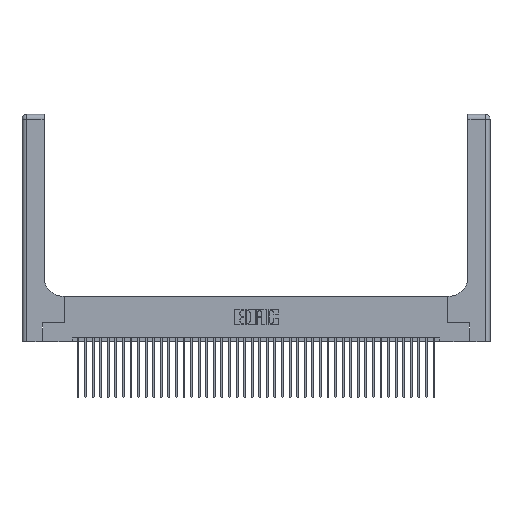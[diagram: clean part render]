
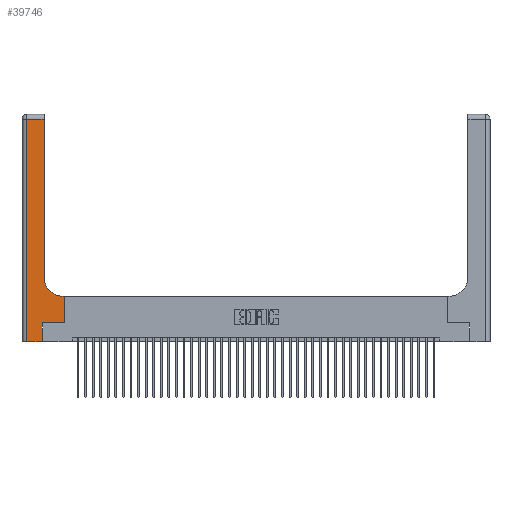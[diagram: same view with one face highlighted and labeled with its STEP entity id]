
A CAD part, top view. The second image highlights one B-rep face of the part: STEP entity #39746.
In plain terms, the highlighted planar face has unit normal (0, 0, 1).
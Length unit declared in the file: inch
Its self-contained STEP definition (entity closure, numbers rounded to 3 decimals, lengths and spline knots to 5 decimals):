
#254 = ORIENTED_EDGE ( 'NONE', *, *, #15014, .T. ) ;
#585 = CARTESIAN_POINT ( 'NONE',  ( 0., 0., 0.37 ) ) ;
#1194 = VERTEX_POINT ( 'NONE', #22436 ) ;
#1436 = LINE ( 'NONE', #27474, #26278 ) ;
#3791 = VERTEX_POINT ( 'NONE', #14060 ) ;
#3934 = CARTESIAN_POINT ( 'NONE',  ( 0.269, 0., 0.37 ) ) ;
#5589 = VERTEX_POINT ( 'NONE', #40948 ) ;
#5886 = VECTOR ( 'NONE', #22582, 39.37008 ) ;
#6122 = VECTOR ( 'NONE', #21281, 39.37008 ) ;
#7618 = AXIS2_PLACEMENT_3D ( 'NONE', #38113, #18554, #41331 ) ;
#7782 = CIRCLE ( 'NONE', #27220, 0.25 ) ;
#8463 = CARTESIAN_POINT ( 'NONE',  ( 0.5585, 0.25, 0.37 ) ) ;
#11759 = ORIENTED_EDGE ( 'NONE', *, *, #21643, .T. ) ;
#11801 = CARTESIAN_POINT ( 'NONE',  ( 0.2915, 0.85, 0.37 ) ) ;
#12279 = LINE ( 'NONE', #29658, #19799 ) ;
#12630 = ORIENTED_EDGE ( 'NONE', *, *, #26330, .T. ) ;
#13741 = EDGE_CURVE ( 'NONE', #40536, #22841, #33933, .T. ) ;
#14060 = CARTESIAN_POINT ( 'NONE',  ( 0.5415, 0.6, 0.37 ) ) ;
#14163 = CARTESIAN_POINT ( 'NONE',  ( 0.5585, 0.6, 0.37 ) ) ;
#14260 = DIRECTION ( 'NONE',  ( 0., 0., -1. ) ) ;
#15014 = EDGE_CURVE ( 'NONE', #21714, #40536, #32266, .T. ) ;
#15228 = CARTESIAN_POINT ( 'NONE',  ( 0.06, 0., 0.37 ) ) ;
#16232 = LINE ( 'NONE', #25360, #40175 ) ;
#16859 = EDGE_CURVE ( 'NONE', #22841, #5589, #12279, .T. ) ;
#17804 = CARTESIAN_POINT ( 'NONE',  ( 0.269, 0.25, 0.37 ) ) ;
#18554 = DIRECTION ( 'NONE',  ( 0., 0., -1. ) ) ;
#18874 = ORIENTED_EDGE ( 'NONE', *, *, #30390, .T. ) ;
#19309 = CARTESIAN_POINT ( 'NONE',  ( 0.2915, 3., 0.37 ) ) ;
#19375 = ORIENTED_EDGE ( 'NONE', *, *, #27619, .T. ) ;
#19799 = VECTOR ( 'NONE', #39519, 39.37008 ) ;
#19962 = DIRECTION ( 'NONE',  ( 1., 0., 0. ) ) ;
#20142 = VERTEX_POINT ( 'NONE', #23522 ) ;
#20660 = ORIENTED_EDGE ( 'NONE', *, *, #16859, .T. ) ;
#21281 = DIRECTION ( 'NONE',  ( 0., 1., 0. ) ) ;
#21643 = EDGE_CURVE ( 'NONE', #5589, #40158, #32021, .T. ) ;
#21714 = VERTEX_POINT ( 'NONE', #15228 ) ;
#22101 = DIRECTION ( 'NONE',  ( -1., 0., 0. ) ) ;
#22436 = CARTESIAN_POINT ( 'NONE',  ( 0.2915, 2.94, 0.37 ) ) ;
#22582 = DIRECTION ( 'NONE',  ( 0., 1., 0. ) ) ;
#22841 = VERTEX_POINT ( 'NONE', #17804 ) ;
#23105 = FACE_OUTER_BOUND ( 'NONE', #34249, .T. ) ;
#23522 = CARTESIAN_POINT ( 'NONE',  ( 0.06, 2.94, 0.37 ) ) ;
#23580 = VECTOR ( 'NONE', #19962, 39.37008 ) ;
#24634 = DIRECTION ( 'NONE',  ( -1., 0., 0. ) ) ;
#24677 = ORIENTED_EDGE ( 'NONE', *, *, #13741, .T. ) ;
#25171 = VECTOR ( 'NONE', #29698, 39.37008 ) ;
#25360 = CARTESIAN_POINT ( 'NONE',  ( 0., 2.94, 0.37 ) ) ;
#26278 = VECTOR ( 'NONE', #37379, 39.37008 ) ;
#26330 = EDGE_CURVE ( 'NONE', #20142, #21714, #1436, .T. ) ;
#27220 = AXIS2_PLACEMENT_3D ( 'NONE', #33746, #14260, #37048 ) ;
#27239 = CARTESIAN_POINT ( 'NONE',  ( 0.2915, 0.6, 0.37 ) ) ;
#27474 = CARTESIAN_POINT ( 'NONE',  ( 0.06, 3., 0.37 ) ) ;
#27619 = EDGE_CURVE ( 'NONE', #40158, #3791, #40970, .T. ) ;
#28560 = EDGE_CURVE ( 'NONE', #36128, #1194, #39459, .T. ) ;
#29658 = CARTESIAN_POINT ( 'NONE',  ( 0.269, 0.25, 0.37 ) ) ;
#29698 = DIRECTION ( 'NONE',  ( 0., 1., 0. ) ) ;
#30390 = EDGE_CURVE ( 'NONE', #3791, #36128, #7782, .T. ) ;
#32021 = LINE ( 'NONE', #8463, #6122 ) ;
#32266 = LINE ( 'NONE', #585, #23580 ) ;
#32859 = EDGE_CURVE ( 'NONE', #1194, #20142, #16232, .T. ) ;
#33746 = CARTESIAN_POINT ( 'NONE',  ( 0.5415, 0.85, 0.37 ) ) ;
#33933 = LINE ( 'NONE', #36171, #25171 ) ;
#34249 = EDGE_LOOP ( 'NONE', ( #34921, #35461, #12630, #254, #24677, #20660, #11759, #19375, #18874 ) ) ;
#34544 = PLANE ( 'NONE',  #7618 ) ;
#34921 = ORIENTED_EDGE ( 'NONE', *, *, #28560, .T. ) ;
#35461 = ORIENTED_EDGE ( 'NONE', *, *, #32859, .T. ) ;
#36128 = VERTEX_POINT ( 'NONE', #11801 ) ;
#36171 = CARTESIAN_POINT ( 'NONE',  ( 0.269, 0., 0.37 ) ) ;
#37048 = DIRECTION ( 'NONE',  ( 1., 0., 0. ) ) ;
#37379 = DIRECTION ( 'NONE',  ( 0., -1., 0. ) ) ;
#38113 = CARTESIAN_POINT ( 'NONE',  ( 0., 3., 0.37 ) ) ;
#39459 = LINE ( 'NONE', #19309, #5886 ) ;
#39519 = DIRECTION ( 'NONE',  ( 1., 0., 0. ) ) ;
#39746 = ADVANCED_FACE ( 'NONE', ( #23105 ), #34544, .F. ) ;
#39963 = VECTOR ( 'NONE', #24634, 39.37008 ) ;
#40158 = VERTEX_POINT ( 'NONE', #14163 ) ;
#40175 = VECTOR ( 'NONE', #22101, 39.37008 ) ;
#40536 = VERTEX_POINT ( 'NONE', #3934 ) ;
#40948 = CARTESIAN_POINT ( 'NONE',  ( 0.5585, 0.25, 0.37 ) ) ;
#40970 = LINE ( 'NONE', #27239, #39963 ) ;
#41331 = DIRECTION ( 'NONE',  ( -1., 0., 0. ) ) ;
